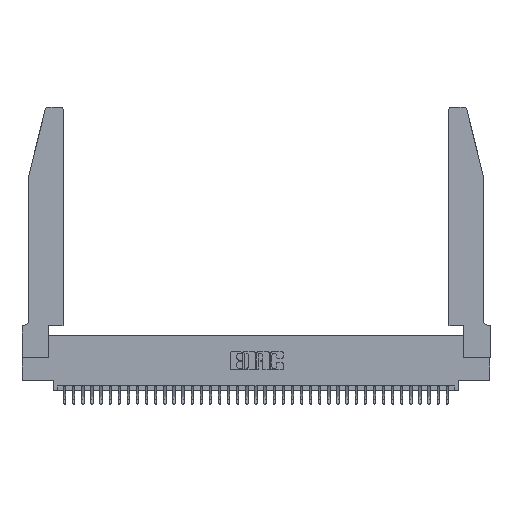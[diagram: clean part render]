
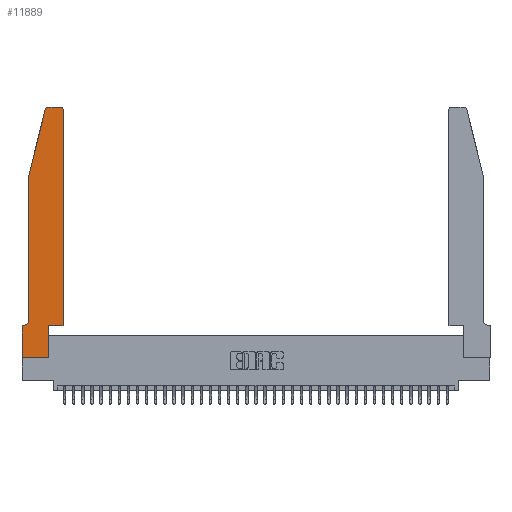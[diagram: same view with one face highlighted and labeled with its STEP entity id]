
A CAD part, top view. The second image highlights one B-rep face of the part: STEP entity #11889.
In plain terms, the highlighted planar face has unit normal (0, 0, 1).
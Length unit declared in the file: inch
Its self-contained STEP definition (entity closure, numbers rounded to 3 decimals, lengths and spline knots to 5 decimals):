
#68 = LINE ( 'NONE', #31306, #24370 ) ;
#876 = ORIENTED_EDGE ( 'NONE', *, *, #17853, .T. ) ;
#2287 = CARTESIAN_POINT ( 'NONE',  ( 0.0755, 2., 0.37 ) ) ;
#3166 = VECTOR ( 'NONE', #14573, 39.37008 ) ;
#3641 = ORIENTED_EDGE ( 'NONE', *, *, #33194, .T. ) ;
#4150 = ORIENTED_EDGE ( 'NONE', *, *, #7418, .T. ) ;
#4543 = CARTESIAN_POINT ( 'NONE',  ( 0.4505, 0.35, 0.37 ) ) ;
#5627 = DIRECTION ( 'NONE',  ( 0., 1., 0. ) ) ;
#5837 = CARTESIAN_POINT ( 'NONE',  ( 0.0755, 2., 0.37 ) ) ;
#6395 = EDGE_CURVE ( 'NONE', #16428, #10715, #6875, .T. ) ;
#6572 = CARTESIAN_POINT ( 'NONE',  ( 0.0055, 0.35, 0.37 ) ) ;
#6875 = LINE ( 'NONE', #5837, #3166 ) ;
#7052 = PLANE ( 'NONE',  #38454 ) ;
#7190 = CARTESIAN_POINT ( 'NONE',  ( 0., 0.35, 0.37 ) ) ;
#7239 = EDGE_LOOP ( 'NONE', ( #37511, #27902, #16561, #29257, #28309, #10242, #3641, #4150, #876, #33819, #27814, #21215 ) ) ;
#7418 = EDGE_CURVE ( 'NONE', #13354, #12219, #8197, .T. ) ;
#8080 = EDGE_CURVE ( 'NONE', #35329, #28726, #22612, .T. ) ;
#8197 = LINE ( 'NONE', #30508, #36770 ) ;
#8253 = VERTEX_POINT ( 'NONE', #6572 ) ;
#9099 = VERTEX_POINT ( 'NONE', #32094 ) ;
#10242 = ORIENTED_EDGE ( 'NONE', *, *, #13853, .T. ) ;
#10715 = VERTEX_POINT ( 'NONE', #17475 ) ;
#11056 = DIRECTION ( 'NONE',  ( -1., 0., 0. ) ) ;
#11218 = DIRECTION ( 'NONE',  ( -1., 0., 0. ) ) ;
#11532 = CIRCLE ( 'NONE', #36446, 0.07 ) ;
#11813 = EDGE_CURVE ( 'NONE', #10715, #8253, #11532, .T. ) ;
#11889 = ADVANCED_FACE ( 'NONE', ( #25078 ), #7052, .T. ) ;
#12219 = VERTEX_POINT ( 'NONE', #29184 ) ;
#12359 = EDGE_CURVE ( 'NONE', #12665, #28555, #21705, .T. ) ;
#12665 = VERTEX_POINT ( 'NONE', #36296 ) ;
#12713 = CIRCLE ( 'NONE', #32955, 0.03 ) ;
#13185 = LINE ( 'NONE', #18192, #20178 ) ;
#13292 = LINE ( 'NONE', #29983, #38100 ) ;
#13354 = VERTEX_POINT ( 'NONE', #26929 ) ;
#13853 = EDGE_CURVE ( 'NONE', #8253, #25481, #13292, .T. ) ;
#14472 = DIRECTION ( 'NONE',  ( 0., 0., -1. ) ) ;
#14573 = DIRECTION ( 'NONE',  ( 0., -1., 0. ) ) ;
#16181 = DIRECTION ( 'NONE',  ( 1., 0., 0. ) ) ;
#16428 = VERTEX_POINT ( 'NONE', #2287 ) ;
#16561 = ORIENTED_EDGE ( 'NONE', *, *, #37044, .T. ) ;
#16836 = CARTESIAN_POINT ( 'NONE',  ( 0.4505, 0.35, 0.37 ) ) ;
#17462 = EDGE_CURVE ( 'NONE', #9099, #22272, #12713, .T. ) ;
#17475 = CARTESIAN_POINT ( 'NONE',  ( 0.0755, 0.42, 0.37 ) ) ;
#17853 = EDGE_CURVE ( 'NONE', #12219, #35329, #68, .T. ) ;
#18192 = CARTESIAN_POINT ( 'NONE',  ( 0., 0., 0.37 ) ) ;
#19489 = DIRECTION ( 'NONE',  ( 0., 1., 0. ) ) ;
#20178 = VECTOR ( 'NONE', #36064, 39.37008 ) ;
#20485 = CARTESIAN_POINT ( 'NONE',  ( 0., 0.35, 0.37 ) ) ;
#21100 = CARTESIAN_POINT ( 'NONE',  ( 0.0755, 2., 0.37 ) ) ;
#21215 = ORIENTED_EDGE ( 'NONE', *, *, #12359, .T. ) ;
#21705 = CIRCLE ( 'NONE', #37692, 0.03 ) ;
#21739 = VECTOR ( 'NONE', #5627, 39.37008 ) ;
#22272 = VERTEX_POINT ( 'NONE', #37783 ) ;
#22612 = LINE ( 'NONE', #4543, #35327 ) ;
#23031 = CARTESIAN_POINT ( 'NONE',  ( 0.2605, 2.75, 0.37 ) ) ;
#23078 = CARTESIAN_POINT ( 'NONE',  ( 0.4205, 2.75, 0.37 ) ) ;
#23233 = LINE ( 'NONE', #23031, #27424 ) ;
#24370 = VECTOR ( 'NONE', #19489, 39.37008 ) ;
#24854 = CARTESIAN_POINT ( 'NONE',  ( 0.4205, 2.72, 0.37 ) ) ;
#25078 = FACE_OUTER_BOUND ( 'NONE', #7239, .T. ) ;
#25481 = VERTEX_POINT ( 'NONE', #20485 ) ;
#26229 = CARTESIAN_POINT ( 'NONE',  ( 0.0055, 0.42, 0.37 ) ) ;
#26689 = DIRECTION ( 'NONE',  ( 1., 0., 0. ) ) ;
#26864 = CARTESIAN_POINT ( 'NONE',  ( 0.4505, 0.35, 0.37 ) ) ;
#26913 = LINE ( 'NONE', #16836, #21739 ) ;
#26929 = CARTESIAN_POINT ( 'NONE',  ( 0., 0., 0.37 ) ) ;
#27424 = VECTOR ( 'NONE', #34996, 39.37008 ) ;
#27814 = ORIENTED_EDGE ( 'NONE', *, *, #36263, .T. ) ;
#27902 = ORIENTED_EDGE ( 'NONE', *, *, #17462, .T. ) ;
#27953 = CARTESIAN_POINT ( 'NONE',  ( 0.284, 2.72, 0.37 ) ) ;
#28309 = ORIENTED_EDGE ( 'NONE', *, *, #11813, .T. ) ;
#28555 = VERTEX_POINT ( 'NONE', #23078 ) ;
#28726 = VERTEX_POINT ( 'NONE', #26864 ) ;
#29184 = CARTESIAN_POINT ( 'NONE',  ( 0.2865, 0., 0.37 ) ) ;
#29257 = ORIENTED_EDGE ( 'NONE', *, *, #6395, .T. ) ;
#29983 = CARTESIAN_POINT ( 'NONE',  ( 0.0755, 0.35, 0.37 ) ) ;
#30508 = CARTESIAN_POINT ( 'NONE',  ( 0., 0., 0.37 ) ) ;
#30638 = DIRECTION ( 'NONE',  ( 1., 0., 0. ) ) ;
#31306 = CARTESIAN_POINT ( 'NONE',  ( 0.2865, 0.35, 0.37 ) ) ;
#31440 = CARTESIAN_POINT ( 'NONE',  ( 0.2865, 0.35, 0.37 ) ) ;
#31559 = VECTOR ( 'NONE', #33200, 39.37008 ) ;
#32094 = CARTESIAN_POINT ( 'NONE',  ( 0.284, 2.75, 0.37 ) ) ;
#32243 = DIRECTION ( 'NONE',  ( 0., 0., 1. ) ) ;
#32955 = AXIS2_PLACEMENT_3D ( 'NONE', #27953, #34036, #34420 ) ;
#33194 = EDGE_CURVE ( 'NONE', #25481, #13354, #13185, .T. ) ;
#33200 = DIRECTION ( 'NONE',  ( -0.239, -0.971, 0. ) ) ;
#33819 = ORIENTED_EDGE ( 'NONE', *, *, #8080, .T. ) ;
#34036 = DIRECTION ( 'NONE',  ( 0., 0., 1. ) ) ;
#34161 = DIRECTION ( 'NONE',  ( 0., 0., 1. ) ) ;
#34420 = DIRECTION ( 'NONE',  ( 1., 0., 0. ) ) ;
#34996 = DIRECTION ( 'NONE',  ( -1., 0., 0. ) ) ;
#35327 = VECTOR ( 'NONE', #37587, 39.37008 ) ;
#35329 = VERTEX_POINT ( 'NONE', #31440 ) ;
#35542 = EDGE_CURVE ( 'NONE', #28555, #9099, #23233, .T. ) ;
#36064 = DIRECTION ( 'NONE',  ( 0., -1., 0. ) ) ;
#36263 = EDGE_CURVE ( 'NONE', #28726, #12665, #26913, .T. ) ;
#36296 = CARTESIAN_POINT ( 'NONE',  ( 0.4505, 2.72, 0.37 ) ) ;
#36446 = AXIS2_PLACEMENT_3D ( 'NONE', #26229, #14472, #11218 ) ;
#36770 = VECTOR ( 'NONE', #30638, 39.37008 ) ;
#37044 = EDGE_CURVE ( 'NONE', #22272, #16428, #37629, .T. ) ;
#37511 = ORIENTED_EDGE ( 'NONE', *, *, #35542, .T. ) ;
#37587 = DIRECTION ( 'NONE',  ( 1., 0., 0. ) ) ;
#37629 = LINE ( 'NONE', #21100, #31559 ) ;
#37692 = AXIS2_PLACEMENT_3D ( 'NONE', #24854, #32243, #26689 ) ;
#37783 = CARTESIAN_POINT ( 'NONE',  ( 0.25487, 2.72718, 0.37 ) ) ;
#38100 = VECTOR ( 'NONE', #11056, 39.37008 ) ;
#38454 = AXIS2_PLACEMENT_3D ( 'NONE', #7190, #34161, #16181 ) ;
